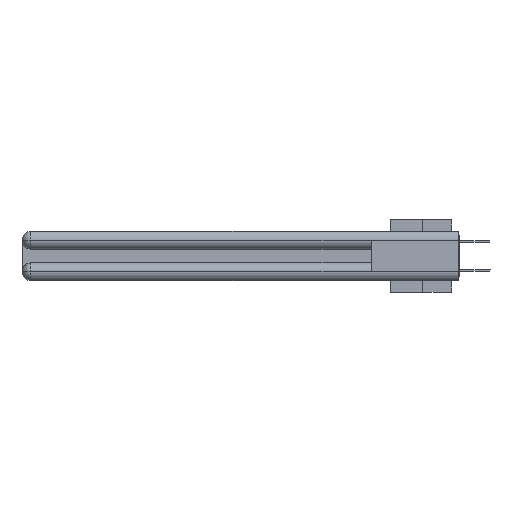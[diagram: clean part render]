
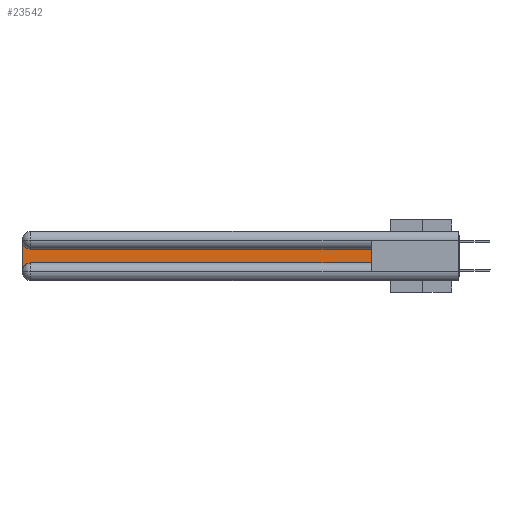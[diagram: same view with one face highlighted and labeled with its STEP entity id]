
A CAD part, left-side view. The second image highlights one B-rep face of the part: STEP entity #23542.
In plain terms, the highlighted planar face has unit normal (-1, 0, 0).
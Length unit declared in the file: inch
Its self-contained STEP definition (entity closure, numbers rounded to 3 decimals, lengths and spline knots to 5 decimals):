
#559 = VECTOR ( 'NONE', #8129, 39.37008 ) ;
#1629 = DIRECTION ( 'NONE',  ( 0., 0., 1. ) ) ;
#1914 = ORIENTED_EDGE ( 'NONE', *, *, #2646, .T. ) ;
#2432 = VERTEX_POINT ( 'NONE', #5010 ) ;
#2646 = EDGE_CURVE ( 'NONE', #14981, #11579, #31948, .T. ) ;
#3359 = CARTESIAN_POINT ( 'NONE',  ( 0.075, 0.6, -0.1225 ) ) ;
#3635 = EDGE_LOOP ( 'NONE', ( #32286, #22483, #13013, #11151, #1914, #29977 ) ) ;
#4378 = EDGE_CURVE ( 'NONE', #11579, #23631, #16493, .T. ) ;
#4757 = CIRCLE ( 'NONE', #9997, 0.06 ) ;
#5010 = CARTESIAN_POINT ( 'NONE',  ( 0.075, 2.94, -0.1225 ) ) ;
#5767 = FACE_OUTER_BOUND ( 'NONE', #3635, .T. ) ;
#6082 = DIRECTION ( 'NONE',  ( 0., 0., -1. ) ) ;
#6469 = DIRECTION ( 'NONE',  ( 1., 0., 0. ) ) ;
#6950 = VERTEX_POINT ( 'NONE', #21102 ) ;
#7274 = VECTOR ( 'NONE', #1629, 39.37008 ) ;
#7680 = LINE ( 'NONE', #24855, #9112 ) ;
#7905 = CARTESIAN_POINT ( 'NONE',  ( 0.075, 3., -0.0625 ) ) ;
#8074 = CIRCLE ( 'NONE', #26354, 0.06 ) ;
#8094 = EDGE_CURVE ( 'NONE', #6950, #14981, #8074, .T. ) ;
#8129 = DIRECTION ( 'NONE',  ( 0., 1., 0. ) ) ;
#9112 = VECTOR ( 'NONE', #17632, 39.37008 ) ;
#9997 = AXIS2_PLACEMENT_3D ( 'NONE', #28389, #6469, #11049 ) ;
#11049 = DIRECTION ( 'NONE',  ( 0., 0., -1. ) ) ;
#11151 = ORIENTED_EDGE ( 'NONE', *, *, #8094, .T. ) ;
#11579 = VERTEX_POINT ( 'NONE', #27204 ) ;
#12929 = AXIS2_PLACEMENT_3D ( 'NONE', #28173, #28486, #6082 ) ;
#13013 = ORIENTED_EDGE ( 'NONE', *, *, #30944, .T. ) ;
#14054 = CARTESIAN_POINT ( 'NONE',  ( 0.075, 0.6, -0.2175 ) ) ;
#14981 = VERTEX_POINT ( 'NONE', #24353 ) ;
#15463 = VECTOR ( 'NONE', #29482, 39.37008 ) ;
#16493 = LINE ( 'NONE', #14054, #7274 ) ;
#17632 = DIRECTION ( 'NONE',  ( 0., 0., -1. ) ) ;
#17690 = EDGE_CURVE ( 'NONE', #23631, #2432, #30504, .T. ) ;
#17738 = EDGE_CURVE ( 'NONE', #2432, #23050, #4757, .T. ) ;
#17867 = CARTESIAN_POINT ( 'NONE',  ( 0.075, 2.94, -0.2775 ) ) ;
#19497 = CARTESIAN_POINT ( 'NONE',  ( 0.075, 0.6, -0.2175 ) ) ;
#21102 = CARTESIAN_POINT ( 'NONE',  ( 0.075, 3., -0.2775 ) ) ;
#22483 = ORIENTED_EDGE ( 'NONE', *, *, #17738, .T. ) ;
#22946 = PLANE ( 'NONE',  #12929 ) ;
#23050 = VERTEX_POINT ( 'NONE', #7905 ) ;
#23542 = ADVANCED_FACE ( 'NONE', ( #5767 ), #22946, .F. ) ;
#23631 = VERTEX_POINT ( 'NONE', #28656 ) ;
#24353 = CARTESIAN_POINT ( 'NONE',  ( 0.075, 2.94, -0.2175 ) ) ;
#24855 = CARTESIAN_POINT ( 'NONE',  ( 0.075, 3., -0.2175 ) ) ;
#25410 = DIRECTION ( 'NONE',  ( 1., 0., 0. ) ) ;
#26354 = AXIS2_PLACEMENT_3D ( 'NONE', #17867, #25410, #26360 ) ;
#26360 = DIRECTION ( 'NONE',  ( 0., 0., -1. ) ) ;
#27204 = CARTESIAN_POINT ( 'NONE',  ( 0.075, 0.6, -0.2175 ) ) ;
#28173 = CARTESIAN_POINT ( 'NONE',  ( 0.075, 3., -0.1225 ) ) ;
#28389 = CARTESIAN_POINT ( 'NONE',  ( 0.075, 2.94, -0.0625 ) ) ;
#28486 = DIRECTION ( 'NONE',  ( 1., 0., 0. ) ) ;
#28656 = CARTESIAN_POINT ( 'NONE',  ( 0.075, 0.6, -0.1225 ) ) ;
#29482 = DIRECTION ( 'NONE',  ( 0., -1., 0. ) ) ;
#29977 = ORIENTED_EDGE ( 'NONE', *, *, #4378, .T. ) ;
#30504 = LINE ( 'NONE', #3359, #559 ) ;
#30944 = EDGE_CURVE ( 'NONE', #23050, #6950, #7680, .T. ) ;
#31948 = LINE ( 'NONE', #19497, #15463 ) ;
#32286 = ORIENTED_EDGE ( 'NONE', *, *, #17690, .T. ) ;
